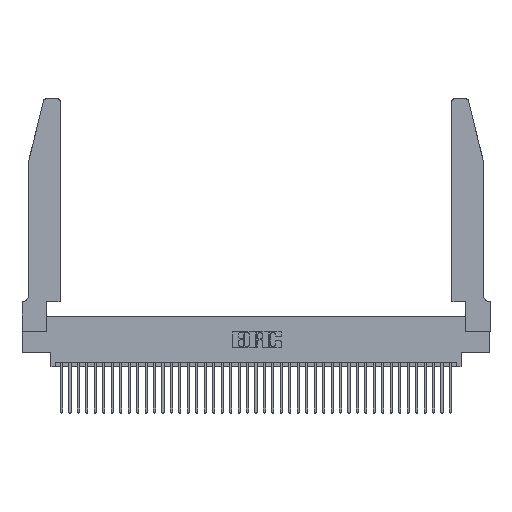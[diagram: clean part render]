
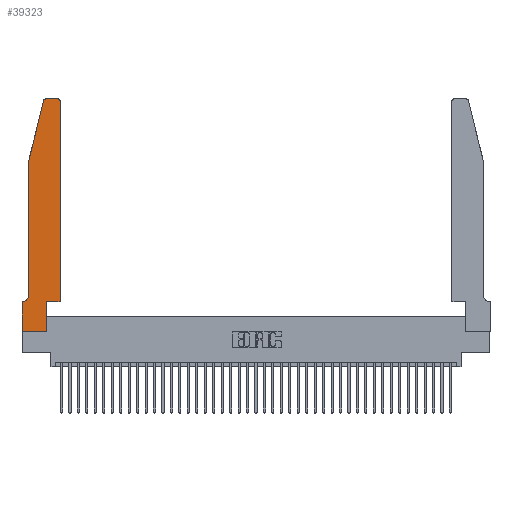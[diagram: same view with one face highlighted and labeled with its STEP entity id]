
A CAD part, top view. The second image highlights one B-rep face of the part: STEP entity #39323.
In plain terms, the highlighted planar face has unit normal (0, 0, 1).
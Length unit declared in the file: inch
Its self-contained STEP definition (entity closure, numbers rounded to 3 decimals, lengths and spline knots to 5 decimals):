
#151 = DIRECTION ( 'NONE',  ( 1., 0., 0. ) ) ;
#550 = CARTESIAN_POINT ( 'NONE',  ( 0., 0.35, 0.37 ) ) ;
#1480 = ORIENTED_EDGE ( 'NONE', *, *, #40875, .T. ) ;
#2477 = AXIS2_PLACEMENT_3D ( 'NONE', #40634, #21891, #2628 ) ;
#2628 = DIRECTION ( 'NONE',  ( -1., 0., 0. ) ) ;
#2827 = VECTOR ( 'NONE', #10476, 39.37008 ) ;
#3493 = CARTESIAN_POINT ( 'NONE',  ( 0.284, 2.75, 0.37 ) ) ;
#3812 = LINE ( 'NONE', #7229, #2827 ) ;
#3824 = EDGE_CURVE ( 'NONE', #13998, #4111, #3812, .T. ) ;
#4111 = VERTEX_POINT ( 'NONE', #15251 ) ;
#4813 = ORIENTED_EDGE ( 'NONE', *, *, #21111, .T. ) ;
#5314 = ORIENTED_EDGE ( 'NONE', *, *, #34186, .T. ) ;
#5762 = VECTOR ( 'NONE', #36839, 39.37008 ) ;
#6394 = VERTEX_POINT ( 'NONE', #36713 ) ;
#7044 = DIRECTION ( 'NONE',  ( 0., 0., 1. ) ) ;
#7229 = CARTESIAN_POINT ( 'NONE',  ( 0.0755, 2., 0.37 ) ) ;
#7428 = DIRECTION ( 'NONE',  ( -1., 0., 0. ) ) ;
#8205 = VECTOR ( 'NONE', #39434, 39.37008 ) ;
#8827 = VECTOR ( 'NONE', #12717, 39.37008 ) ;
#10476 = DIRECTION ( 'NONE',  ( 0., -1., 0. ) ) ;
#10545 = CARTESIAN_POINT ( 'NONE',  ( 0.2605, 2.75, 0.37 ) ) ;
#10939 = ORIENTED_EDGE ( 'NONE', *, *, #37760, .T. ) ;
#11573 = CARTESIAN_POINT ( 'NONE',  ( 0.0755, 0.35, 0.37 ) ) ;
#11681 = CARTESIAN_POINT ( 'NONE',  ( 0.0755, 2., 0.37 ) ) ;
#11873 = EDGE_LOOP ( 'NONE', ( #5314, #4813, #24895, #22426, #21960, #24931, #10939, #32789, #31356, #1480, #30979, #18606 ) ) ;
#11931 = VERTEX_POINT ( 'NONE', #32517 ) ;
#12448 = EDGE_CURVE ( 'NONE', #28033, #13998, #23906, .T. ) ;
#12717 = DIRECTION ( 'NONE',  ( 0., 1., 0. ) ) ;
#12960 = AXIS2_PLACEMENT_3D ( 'NONE', #38245, #19405, #151 ) ;
#13998 = VERTEX_POINT ( 'NONE', #15868 ) ;
#14254 = CARTESIAN_POINT ( 'NONE',  ( 0.2865, 0., 0.37 ) ) ;
#14895 = DIRECTION ( 'NONE',  ( -0.239, -0.971, 0. ) ) ;
#15251 = CARTESIAN_POINT ( 'NONE',  ( 0.0755, 0.42, 0.37 ) ) ;
#15868 = CARTESIAN_POINT ( 'NONE',  ( 0.0755, 2., 0.37 ) ) ;
#16750 = CARTESIAN_POINT ( 'NONE',  ( 0.4505, 0.35, 0.37 ) ) ;
#17767 = CARTESIAN_POINT ( 'NONE',  ( 0.284, 2.72, 0.37 ) ) ;
#18186 = DIRECTION ( 'NONE',  ( 1., 0., 0. ) ) ;
#18606 = ORIENTED_EDGE ( 'NONE', *, *, #24053, .T. ) ;
#19405 = DIRECTION ( 'NONE',  ( 0., 0., 1. ) ) ;
#19555 = CARTESIAN_POINT ( 'NONE',  ( 0.4205, 2.75, 0.37 ) ) ;
#20291 = CARTESIAN_POINT ( 'NONE',  ( 0.0055, 0.35, 0.37 ) ) ;
#20624 = CARTESIAN_POINT ( 'NONE',  ( 0.4505, 0.35, 0.37 ) ) ;
#20983 = DIRECTION ( 'NONE',  ( 1., 0., 0. ) ) ;
#21111 = EDGE_CURVE ( 'NONE', #26623, #28033, #31783, .T. ) ;
#21891 = DIRECTION ( 'NONE',  ( 0., 0., -1. ) ) ;
#21960 = ORIENTED_EDGE ( 'NONE', *, *, #34540, .T. ) ;
#22248 = VECTOR ( 'NONE', #30958, 39.37008 ) ;
#22426 = ORIENTED_EDGE ( 'NONE', *, *, #3824, .T. ) ;
#22507 = CARTESIAN_POINT ( 'NONE',  ( 0.4505, 0.35, 0.37 ) ) ;
#22819 = LINE ( 'NONE', #11573, #5762 ) ;
#22895 = VECTOR ( 'NONE', #14895, 39.37008 ) ;
#23509 = CIRCLE ( 'NONE', #2477, 0.07 ) ;
#23555 = VERTEX_POINT ( 'NONE', #14254 ) ;
#23906 = LINE ( 'NONE', #11681, #22895 ) ;
#24053 = EDGE_CURVE ( 'NONE', #11931, #31000, #26212, .T. ) ;
#24353 = CARTESIAN_POINT ( 'NONE',  ( 0.2865, 0.35, 0.37 ) ) ;
#24553 = LINE ( 'NONE', #22507, #39214 ) ;
#24619 = CARTESIAN_POINT ( 'NONE',  ( 0., 0., 0.37 ) ) ;
#24895 = ORIENTED_EDGE ( 'NONE', *, *, #12448, .T. ) ;
#24931 = ORIENTED_EDGE ( 'NONE', *, *, #29348, .T. ) ;
#25240 = LINE ( 'NONE', #20624, #8205 ) ;
#25632 = EDGE_CURVE ( 'NONE', #6394, #23555, #26055, .T. ) ;
#26055 = LINE ( 'NONE', #40181, #33400 ) ;
#26212 = CIRCLE ( 'NONE', #12960, 0.03 ) ;
#26216 = PLANE ( 'NONE',  #41092 ) ;
#26623 = VERTEX_POINT ( 'NONE', #3493 ) ;
#26799 = CARTESIAN_POINT ( 'NONE',  ( 0., 0.35, 0.37 ) ) ;
#26829 = CARTESIAN_POINT ( 'NONE',  ( 0.25487, 2.72718, 0.37 ) ) ;
#28033 = VERTEX_POINT ( 'NONE', #26829 ) ;
#28179 = DIRECTION ( 'NONE',  ( 1., 0., 0. ) ) ;
#28870 = EDGE_CURVE ( 'NONE', #23555, #32492, #39504, .T. ) ;
#29348 = EDGE_CURVE ( 'NONE', #34747, #38800, #22819, .T. ) ;
#29370 = DIRECTION ( 'NONE',  ( 1., 0., 0. ) ) ;
#29904 = EDGE_CURVE ( 'NONE', #38083, #11931, #25240, .T. ) ;
#30388 = LINE ( 'NONE', #10545, #36689 ) ;
#30636 = LINE ( 'NONE', #24619, #22248 ) ;
#30958 = DIRECTION ( 'NONE',  ( 0., -1., 0. ) ) ;
#30979 = ORIENTED_EDGE ( 'NONE', *, *, #29904, .T. ) ;
#31000 = VERTEX_POINT ( 'NONE', #19555 ) ;
#31356 = ORIENTED_EDGE ( 'NONE', *, *, #28870, .T. ) ;
#31708 = CARTESIAN_POINT ( 'NONE',  ( 0.2865, 0.35, 0.37 ) ) ;
#31783 = CIRCLE ( 'NONE', #34877, 0.03 ) ;
#32492 = VERTEX_POINT ( 'NONE', #24353 ) ;
#32517 = CARTESIAN_POINT ( 'NONE',  ( 0.4505, 2.72, 0.37 ) ) ;
#32789 = ORIENTED_EDGE ( 'NONE', *, *, #25632, .T. ) ;
#33400 = VECTOR ( 'NONE', #18186, 39.37008 ) ;
#33909 = FACE_OUTER_BOUND ( 'NONE', #11873, .T. ) ;
#34186 = EDGE_CURVE ( 'NONE', #31000, #26623, #30388, .T. ) ;
#34540 = EDGE_CURVE ( 'NONE', #4111, #34747, #23509, .T. ) ;
#34747 = VERTEX_POINT ( 'NONE', #20291 ) ;
#34877 = AXIS2_PLACEMENT_3D ( 'NONE', #17767, #39773, #20983 ) ;
#36689 = VECTOR ( 'NONE', #7428, 39.37008 ) ;
#36713 = CARTESIAN_POINT ( 'NONE',  ( 0., 0., 0.37 ) ) ;
#36839 = DIRECTION ( 'NONE',  ( -1., 0., 0. ) ) ;
#37760 = EDGE_CURVE ( 'NONE', #38800, #6394, #30636, .T. ) ;
#38083 = VERTEX_POINT ( 'NONE', #16750 ) ;
#38245 = CARTESIAN_POINT ( 'NONE',  ( 0.4205, 2.72, 0.37 ) ) ;
#38800 = VERTEX_POINT ( 'NONE', #26799 ) ;
#39214 = VECTOR ( 'NONE', #28179, 39.37008 ) ;
#39323 = ADVANCED_FACE ( 'NONE', ( #33909 ), #26216, .T. ) ;
#39434 = DIRECTION ( 'NONE',  ( 0., 1., 0. ) ) ;
#39504 = LINE ( 'NONE', #31708, #8827 ) ;
#39773 = DIRECTION ( 'NONE',  ( 0., 0., 1. ) ) ;
#40181 = CARTESIAN_POINT ( 'NONE',  ( 0., 0., 0.37 ) ) ;
#40634 = CARTESIAN_POINT ( 'NONE',  ( 0.0055, 0.42, 0.37 ) ) ;
#40875 = EDGE_CURVE ( 'NONE', #32492, #38083, #24553, .T. ) ;
#41092 = AXIS2_PLACEMENT_3D ( 'NONE', #550, #7044, #29370 ) ;
